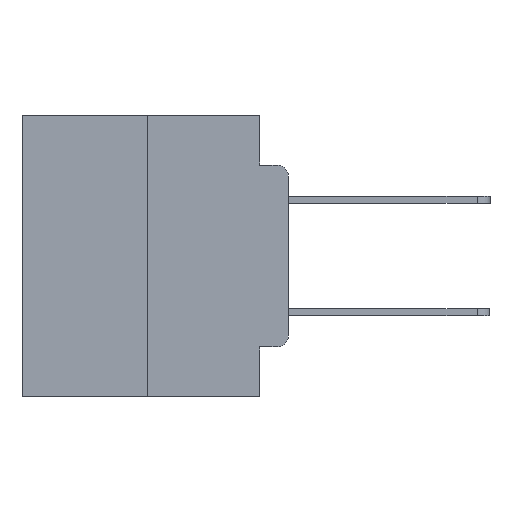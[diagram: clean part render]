
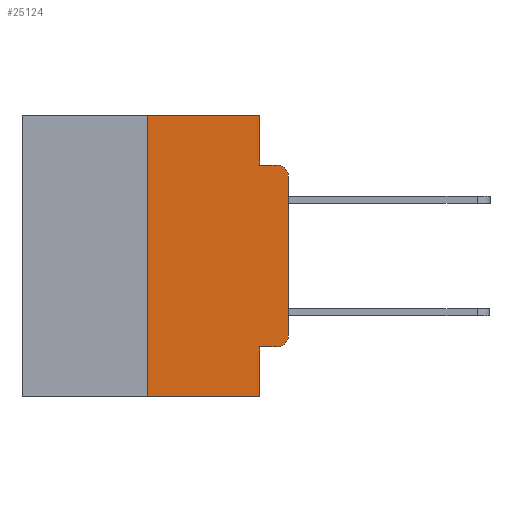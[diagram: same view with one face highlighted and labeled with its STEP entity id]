
A CAD part, left-side view. The second image highlights one B-rep face of the part: STEP entity #25124.
In plain terms, the highlighted planar face has unit normal (-1, 0, 0).
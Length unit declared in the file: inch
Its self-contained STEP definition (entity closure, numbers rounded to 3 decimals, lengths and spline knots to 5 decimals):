
#150 = CARTESIAN_POINT ( 'NONE',  ( 0., 0., -0.1085 ) ) ;
#216 = EDGE_CURVE ( 'NONE', #25857, #24096, #25539, .T. ) ;
#400 = CARTESIAN_POINT ( 'NONE',  ( 0., 0.051, 0. ) ) ;
#610 = EDGE_CURVE ( 'NONE', #8162, #24096, #15925, .T. ) ;
#765 = ORIENTED_EDGE ( 'NONE', *, *, #27305, .F. ) ;
#990 = EDGE_CURVE ( 'NONE', #25857, #8000, #1872, .T. ) ;
#1264 = AXIS2_PLACEMENT_3D ( 'NONE', #15056, #23672, #10801 ) ;
#1541 = LINE ( 'NONE', #11715, #23969 ) ;
#1872 = LINE ( 'NONE', #26659, #18597 ) ;
#2221 = CARTESIAN_POINT ( 'NONE',  ( 0., 0.051, -0.0885 ) ) ;
#2267 = DIRECTION ( 'NONE',  ( 0., 0., 1. ) ) ;
#2423 = CARTESIAN_POINT ( 'NONE',  ( 0., 0.051, -0.5 ) ) ;
#3361 = DIRECTION ( 'NONE',  ( 0., 0., -1. ) ) ;
#3455 = LINE ( 'NONE', #8261, #8611 ) ;
#3702 = ORIENTED_EDGE ( 'NONE', *, *, #610, .F. ) ;
#4462 = CARTESIAN_POINT ( 'NONE',  ( 0., 0.02, -0.1085 ) ) ;
#5050 = VECTOR ( 'NONE', #2267, 39.37008 ) ;
#5268 = CARTESIAN_POINT ( 'NONE',  ( 0., 0.051, -0.4115 ) ) ;
#5514 = CARTESIAN_POINT ( 'NONE',  ( 0., 0., -0.3915 ) ) ;
#6362 = CARTESIAN_POINT ( 'NONE',  ( 0., 0.051, 0. ) ) ;
#6677 = DIRECTION ( 'NONE',  ( 0., -1., 0. ) ) ;
#6680 = DIRECTION ( 'NONE',  ( 0., 0., -1. ) ) ;
#6853 = DIRECTION ( 'NONE',  ( -1., 0., 0. ) ) ;
#7763 = ORIENTED_EDGE ( 'NONE', *, *, #27824, .F. ) ;
#7849 = CIRCLE ( 'NONE', #12481, 0.02 ) ;
#8000 = VERTEX_POINT ( 'NONE', #24132 ) ;
#8024 = CIRCLE ( 'NONE', #25778, 0.02 ) ;
#8162 = VERTEX_POINT ( 'NONE', #5268 ) ;
#8261 = CARTESIAN_POINT ( 'NONE',  ( 0., 0.473, 0. ) ) ;
#8308 = CARTESIAN_POINT ( 'NONE',  ( 0., 0.051, -0.0885 ) ) ;
#8417 = VERTEX_POINT ( 'NONE', #8308 ) ;
#8568 = EDGE_CURVE ( 'NONE', #22528, #18973, #7849, .T. ) ;
#8611 = VECTOR ( 'NONE', #19013, 39.37008 ) ;
#8644 = PLANE ( 'NONE',  #1264 ) ;
#9240 = EDGE_CURVE ( 'NONE', #8162, #19184, #1541, .T. ) ;
#9706 = FACE_OUTER_BOUND ( 'NONE', #17242, .T. ) ;
#10160 = VECTOR ( 'NONE', #3361, 39.37008 ) ;
#10615 = VECTOR ( 'NONE', #26416, 39.37008 ) ;
#10801 = DIRECTION ( 'NONE',  ( 0., 0., -1. ) ) ;
#10842 = ORIENTED_EDGE ( 'NONE', *, *, #216, .T. ) ;
#10871 = ORIENTED_EDGE ( 'NONE', *, *, #9240, .T. ) ;
#11058 = CARTESIAN_POINT ( 'NONE',  ( 0., 0.25, -0.5 ) ) ;
#11488 = EDGE_CURVE ( 'NONE', #19184, #24317, #8024, .T. ) ;
#11715 = CARTESIAN_POINT ( 'NONE',  ( 0., 0.051, -0.4115 ) ) ;
#12481 = AXIS2_PLACEMENT_3D ( 'NONE', #4462, #19613, #6680 ) ;
#14325 = LINE ( 'NONE', #2221, #25013 ) ;
#14594 = VECTOR ( 'NONE', #18278, 39.37008 ) ;
#15056 = CARTESIAN_POINT ( 'NONE',  ( 0., 0.473, 0. ) ) ;
#15143 = EDGE_CURVE ( 'NONE', #24317, #22528, #16597, .T. ) ;
#15925 = LINE ( 'NONE', #6362, #10160 ) ;
#16597 = LINE ( 'NONE', #17529, #5050 ) ;
#17242 = EDGE_LOOP ( 'NONE', ( #21547, #24252, #7763, #765, #18922, #19264, #10842, #3702, #10871, #23646 ) ) ;
#17529 = CARTESIAN_POINT ( 'NONE',  ( 0., 0., 0. ) ) ;
#18224 = DIRECTION ( 'NONE',  ( 0., -1., 0. ) ) ;
#18278 = DIRECTION ( 'NONE',  ( 0., -1., 0. ) ) ;
#18597 = VECTOR ( 'NONE', #26633, 39.37008 ) ;
#18700 = CARTESIAN_POINT ( 'NONE',  ( 0., 0.473, -0.5 ) ) ;
#18922 = ORIENTED_EDGE ( 'NONE', *, *, #21103, .F. ) ;
#18973 = VERTEX_POINT ( 'NONE', #22291 ) ;
#19013 = DIRECTION ( 'NONE',  ( 0., -1., 0. ) ) ;
#19184 = VERTEX_POINT ( 'NONE', #23022 ) ;
#19264 = ORIENTED_EDGE ( 'NONE', *, *, #990, .F. ) ;
#19613 = DIRECTION ( 'NONE',  ( -1., 0., 0. ) ) ;
#19785 = CARTESIAN_POINT ( 'NONE',  ( 0., 0.02, -0.3915 ) ) ;
#21103 = EDGE_CURVE ( 'NONE', #8000, #22772, #3455, .T. ) ;
#21547 = ORIENTED_EDGE ( 'NONE', *, *, #15143, .T. ) ;
#21918 = DIRECTION ( 'NONE',  ( 0., 0., -1. ) ) ;
#22291 = CARTESIAN_POINT ( 'NONE',  ( 0., 0.02, -0.0885 ) ) ;
#22528 = VERTEX_POINT ( 'NONE', #150 ) ;
#22763 = CARTESIAN_POINT ( 'NONE',  ( 0., 0.051, 0. ) ) ;
#22772 = VERTEX_POINT ( 'NONE', #22763 ) ;
#23022 = CARTESIAN_POINT ( 'NONE',  ( 0., 0.02, -0.4115 ) ) ;
#23646 = ORIENTED_EDGE ( 'NONE', *, *, #11488, .T. ) ;
#23672 = DIRECTION ( 'NONE',  ( 1., 0., 0. ) ) ;
#23969 = VECTOR ( 'NONE', #18224, 39.37008 ) ;
#24096 = VERTEX_POINT ( 'NONE', #2423 ) ;
#24132 = CARTESIAN_POINT ( 'NONE',  ( 0., 0.25, 0. ) ) ;
#24252 = ORIENTED_EDGE ( 'NONE', *, *, #8568, .T. ) ;
#24317 = VERTEX_POINT ( 'NONE', #5514 ) ;
#25013 = VECTOR ( 'NONE', #6677, 39.37008 ) ;
#25124 = ADVANCED_FACE ( 'NONE', ( #9706 ), #8644, .F. ) ;
#25539 = LINE ( 'NONE', #18700, #14594 ) ;
#25778 = AXIS2_PLACEMENT_3D ( 'NONE', #19785, #6853, #21918 ) ;
#25857 = VERTEX_POINT ( 'NONE', #11058 ) ;
#26416 = DIRECTION ( 'NONE',  ( 0., 0., -1. ) ) ;
#26633 = DIRECTION ( 'NONE',  ( 0., 0., 1. ) ) ;
#26659 = CARTESIAN_POINT ( 'NONE',  ( 0., 0.25, 0. ) ) ;
#27305 = EDGE_CURVE ( 'NONE', #22772, #8417, #27700, .T. ) ;
#27700 = LINE ( 'NONE', #400, #10615 ) ;
#27824 = EDGE_CURVE ( 'NONE', #8417, #18973, #14325, .T. ) ;
